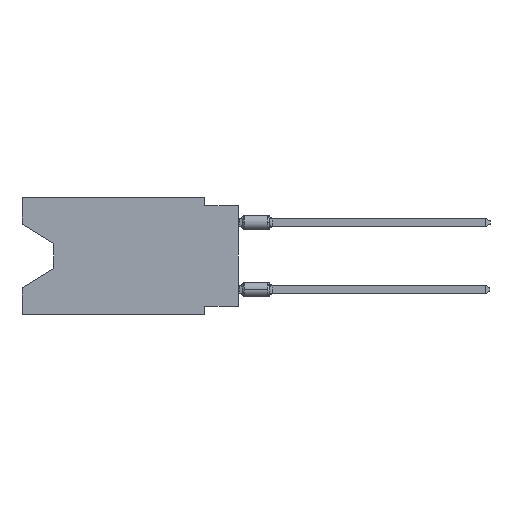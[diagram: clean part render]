
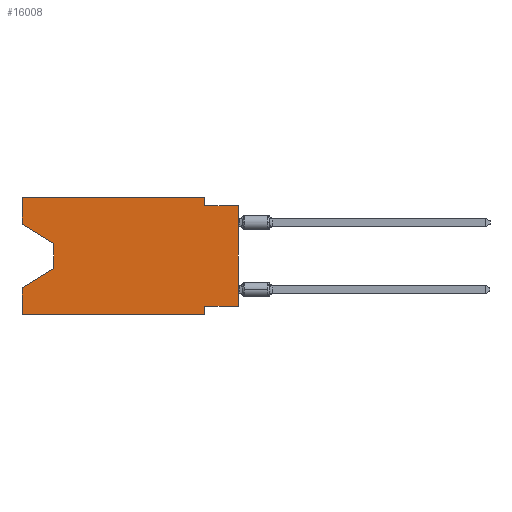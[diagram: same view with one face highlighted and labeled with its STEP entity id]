
A CAD part, left-side view. The second image highlights one B-rep face of the part: STEP entity #16008.
In plain terms, the highlighted planar face has unit normal (-1, 0, 0).
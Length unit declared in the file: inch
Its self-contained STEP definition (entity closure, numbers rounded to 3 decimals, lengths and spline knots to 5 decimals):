
#86 = CARTESIAN_POINT ( 'NONE',  ( 0., 0.645, -0.35 ) ) ;
#181 = VECTOR ( 'NONE', #3519, 39.37008 ) ;
#287 = DIRECTION ( 'NONE',  ( 0., 0., -1. ) ) ;
#340 = VERTEX_POINT ( 'NONE', #10777 ) ;
#472 = CARTESIAN_POINT ( 'NONE',  ( 0., 0.645, -0.08025 ) ) ;
#906 = VERTEX_POINT ( 'NONE', #17837 ) ;
#931 = VECTOR ( 'NONE', #10046, 39.37008 ) ;
#1007 = CARTESIAN_POINT ( 'NONE',  ( 0., 0.1, 0. ) ) ;
#1023 = ORIENTED_EDGE ( 'NONE', *, *, #12648, .T. ) ;
#1210 = VECTOR ( 'NONE', #287, 39.37008 ) ;
#1475 = CARTESIAN_POINT ( 'NONE',  ( 0., 0., -0.325 ) ) ;
#1620 = LINE ( 'NONE', #8469, #17557 ) ;
#1874 = CARTESIAN_POINT ( 'NONE',  ( 0., 0., -0.025 ) ) ;
#2055 = LINE ( 'NONE', #10792, #6136 ) ;
#2203 = VERTEX_POINT ( 'NONE', #3062 ) ;
#2620 = CARTESIAN_POINT ( 'NONE',  ( 0., 0.645, 0. ) ) ;
#2746 = EDGE_CURVE ( 'NONE', #10571, #19809, #3345, .T. ) ;
#2795 = ORIENTED_EDGE ( 'NONE', *, *, #2746, .T. ) ;
#3054 = VECTOR ( 'NONE', #21302, 39.37008 ) ;
#3062 = CARTESIAN_POINT ( 'NONE',  ( 0., 0.55, -0.212 ) ) ;
#3087 = LINE ( 'NONE', #21514, #3054 ) ;
#3345 = LINE ( 'NONE', #86, #4640 ) ;
#3435 = DIRECTION ( 'NONE',  ( 0., 1., 0. ) ) ;
#3448 = LINE ( 'NONE', #14805, #9448 ) ;
#3519 = DIRECTION ( 'NONE',  ( 0., 0., -1. ) ) ;
#3531 = EDGE_CURVE ( 'NONE', #9594, #4197, #1620, .T. ) ;
#4046 = ORIENTED_EDGE ( 'NONE', *, *, #21354, .F. ) ;
#4062 = ORIENTED_EDGE ( 'NONE', *, *, #12266, .T. ) ;
#4084 = EDGE_CURVE ( 'NONE', #4197, #8379, #14124, .T. ) ;
#4197 = VERTEX_POINT ( 'NONE', #10417 ) ;
#4365 = EDGE_CURVE ( 'NONE', #8379, #906, #5469, .T. ) ;
#4640 = VECTOR ( 'NONE', #8794, 39.37008 ) ;
#5172 = DIRECTION ( 'NONE',  ( 0., 0., -1. ) ) ;
#5373 = LINE ( 'NONE', #472, #20787 ) ;
#5427 = CARTESIAN_POINT ( 'NONE',  ( 0., 0., -0.325 ) ) ;
#5469 = LINE ( 'NONE', #20186, #931 ) ;
#6136 = VECTOR ( 'NONE', #20496, 39.37008 ) ;
#6493 = VERTEX_POINT ( 'NONE', #1874 ) ;
#6765 = EDGE_CURVE ( 'NONE', #16696, #19809, #18711, .T. ) ;
#6783 = PLANE ( 'NONE',  #15875 ) ;
#7020 = CARTESIAN_POINT ( 'NONE',  ( 0., 0.1, -0.35 ) ) ;
#7140 = ORIENTED_EDGE ( 'NONE', *, *, #10784, .F. ) ;
#8379 = VERTEX_POINT ( 'NONE', #1007 ) ;
#8469 = CARTESIAN_POINT ( 'NONE',  ( 0., 0.645, 0. ) ) ;
#8794 = DIRECTION ( 'NONE',  ( 0., -1., 0. ) ) ;
#8914 = VECTOR ( 'NONE', #20665, 39.37008 ) ;
#9144 = VERTEX_POINT ( 'NONE', #5427 ) ;
#9294 = DIRECTION ( 'NONE',  ( 0., 0., 1. ) ) ;
#9448 = VECTOR ( 'NONE', #11311, 39.37008 ) ;
#9594 = VERTEX_POINT ( 'NONE', #12341 ) ;
#10046 = DIRECTION ( 'NONE',  ( 0., 0., -1. ) ) ;
#10067 = LINE ( 'NONE', #21413, #181 ) ;
#10085 = LINE ( 'NONE', #1475, #21422 ) ;
#10417 = CARTESIAN_POINT ( 'NONE',  ( 0., 0.645, 0. ) ) ;
#10571 = VERTEX_POINT ( 'NONE', #14476 ) ;
#10777 = CARTESIAN_POINT ( 'NONE',  ( 0., 0.645, -0.26975 ) ) ;
#10784 = EDGE_CURVE ( 'NONE', #10571, #340, #17572, .T. ) ;
#10792 = CARTESIAN_POINT ( 'NONE',  ( 0., 0., 0. ) ) ;
#11054 = CARTESIAN_POINT ( 'NONE',  ( 0., 0.1, -0.325 ) ) ;
#11056 = ORIENTED_EDGE ( 'NONE', *, *, #3531, .F. ) ;
#11223 = EDGE_CURVE ( 'NONE', #2203, #340, #3448, .T. ) ;
#11311 = DIRECTION ( 'NONE',  ( 0., 0.855, -0.519 ) ) ;
#11476 = ORIENTED_EDGE ( 'NONE', *, *, #11223, .T. ) ;
#11965 = DIRECTION ( 'NONE',  ( 0., 0., 1. ) ) ;
#12266 = EDGE_CURVE ( 'NONE', #9144, #6493, #2055, .T. ) ;
#12323 = ORIENTED_EDGE ( 'NONE', *, *, #15967, .T. ) ;
#12341 = CARTESIAN_POINT ( 'NONE',  ( 0., 0.645, -0.08025 ) ) ;
#12648 = EDGE_CURVE ( 'NONE', #9594, #16742, #5373, .T. ) ;
#12968 = CARTESIAN_POINT ( 'NONE',  ( 0., 0.1, -0.35 ) ) ;
#13560 = FACE_OUTER_BOUND ( 'NONE', #18405, .T. ) ;
#14124 = LINE ( 'NONE', #17067, #8914 ) ;
#14476 = CARTESIAN_POINT ( 'NONE',  ( 0., 0.645, -0.35 ) ) ;
#14805 = CARTESIAN_POINT ( 'NONE',  ( 0., 0.55, -0.212 ) ) ;
#15648 = DIRECTION ( 'NONE',  ( 0., -0.855, -0.519 ) ) ;
#15875 = AXIS2_PLACEMENT_3D ( 'NONE', #18149, #20100, #5172 ) ;
#15967 = EDGE_CURVE ( 'NONE', #16742, #2203, #10067, .T. ) ;
#16008 = ADVANCED_FACE ( 'NONE', ( #13560 ), #6783, .F. ) ;
#16042 = ORIENTED_EDGE ( 'NONE', *, *, #6765, .F. ) ;
#16696 = VERTEX_POINT ( 'NONE', #11054 ) ;
#16742 = VERTEX_POINT ( 'NONE', #19552 ) ;
#17067 = CARTESIAN_POINT ( 'NONE',  ( 0., 0.645, 0. ) ) ;
#17557 = VECTOR ( 'NONE', #11965, 39.37008 ) ;
#17572 = LINE ( 'NONE', #2620, #20240 ) ;
#17837 = CARTESIAN_POINT ( 'NONE',  ( 0., 0.1, -0.025 ) ) ;
#18149 = CARTESIAN_POINT ( 'NONE',  ( 0., 0.645, 0. ) ) ;
#18405 = EDGE_LOOP ( 'NONE', ( #1023, #12323, #11476, #7140, #2795, #16042, #20852, #4062, #4046, #19545, #21233, #11056 ) ) ;
#18711 = LINE ( 'NONE', #7020, #1210 ) ;
#18864 = EDGE_CURVE ( 'NONE', #9144, #16696, #10085, .T. ) ;
#19545 = ORIENTED_EDGE ( 'NONE', *, *, #4365, .F. ) ;
#19552 = CARTESIAN_POINT ( 'NONE',  ( 0., 0.55, -0.138 ) ) ;
#19809 = VERTEX_POINT ( 'NONE', #12968 ) ;
#20100 = DIRECTION ( 'NONE',  ( 1., 0., 0. ) ) ;
#20186 = CARTESIAN_POINT ( 'NONE',  ( 0., 0.1, 0. ) ) ;
#20240 = VECTOR ( 'NONE', #9294, 39.37008 ) ;
#20496 = DIRECTION ( 'NONE',  ( 0., 0., 1. ) ) ;
#20665 = DIRECTION ( 'NONE',  ( 0., -1., 0. ) ) ;
#20787 = VECTOR ( 'NONE', #15648, 39.37008 ) ;
#20852 = ORIENTED_EDGE ( 'NONE', *, *, #18864, .F. ) ;
#21233 = ORIENTED_EDGE ( 'NONE', *, *, #4084, .F. ) ;
#21302 = DIRECTION ( 'NONE',  ( 0., -1., 0. ) ) ;
#21354 = EDGE_CURVE ( 'NONE', #906, #6493, #3087, .T. ) ;
#21413 = CARTESIAN_POINT ( 'NONE',  ( 0., 0.55, -0.138 ) ) ;
#21422 = VECTOR ( 'NONE', #3435, 39.37008 ) ;
#21514 = CARTESIAN_POINT ( 'NONE',  ( 0., 0., -0.025 ) ) ;
